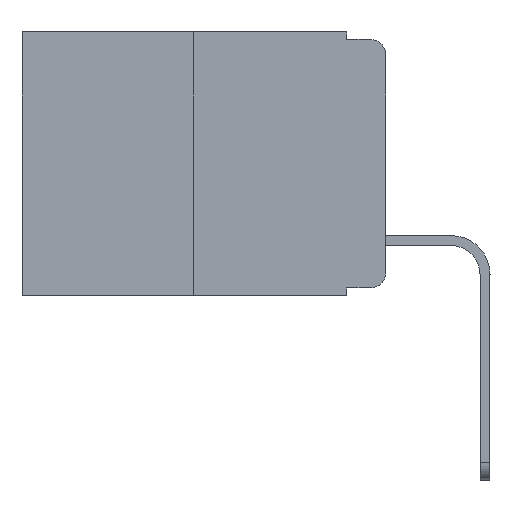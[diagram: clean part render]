
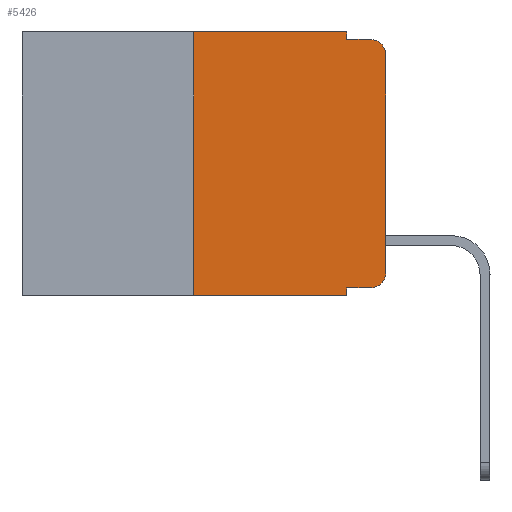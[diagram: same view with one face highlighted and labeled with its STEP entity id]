
A CAD part, left-side view. The second image highlights one B-rep face of the part: STEP entity #5426.
In plain terms, the highlighted planar face has unit normal (-1, 0, 0).
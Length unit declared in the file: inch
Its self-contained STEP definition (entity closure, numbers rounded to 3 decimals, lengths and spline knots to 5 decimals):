
#352 = VERTEX_POINT ( 'NONE', #11392 ) ;
#611 = DIRECTION ( 'NONE',  ( 0., 0., -1. ) ) ;
#621 = EDGE_CURVE ( 'NONE', #10920, #8780, #8117, .T. ) ;
#661 = VECTOR ( 'NONE', #7831, 39.37008 ) ;
#679 = DIRECTION ( 'NONE',  ( 0., 0., -1. ) ) ;
#729 = LINE ( 'NONE', #7810, #7426 ) ;
#863 = DIRECTION ( 'NONE',  ( 0., 0., -1. ) ) ;
#1055 = VERTEX_POINT ( 'NONE', #1663 ) ;
#1110 = ORIENTED_EDGE ( 'NONE', *, *, #11555, .T. ) ;
#1225 = CARTESIAN_POINT ( 'NONE',  ( 0., 0.473, 0. ) ) ;
#1227 = LINE ( 'NONE', #2138, #4111 ) ;
#1252 = ORIENTED_EDGE ( 'NONE', *, *, #7644, .T. ) ;
#1360 = ORIENTED_EDGE ( 'NONE', *, *, #11955, .F. ) ;
#1390 = CIRCLE ( 'NONE', #7680, 0.02 ) ;
#1627 = VECTOR ( 'NONE', #9238, 39.37008 ) ;
#1663 = CARTESIAN_POINT ( 'NONE',  ( 0., 0., -0.03 ) ) ;
#1911 = EDGE_CURVE ( 'NONE', #1055, #9202, #5476, .T. ) ;
#2065 = DIRECTION ( 'NONE',  ( 0., 0., 1. ) ) ;
#2138 = CARTESIAN_POINT ( 'NONE',  ( 0., 0., 0. ) ) ;
#2161 = CARTESIAN_POINT ( 'NONE',  ( 0., 0.02, -0.01 ) ) ;
#2616 = ORIENTED_EDGE ( 'NONE', *, *, #5266, .F. ) ;
#2646 = LINE ( 'NONE', #10412, #11931 ) ;
#3021 = PLANE ( 'NONE',  #4614 ) ;
#3123 = FACE_OUTER_BOUND ( 'NONE', #6134, .T. ) ;
#3201 = CARTESIAN_POINT ( 'NONE',  ( 0., 0.02, -0.333 ) ) ;
#3564 = CARTESIAN_POINT ( 'NONE',  ( 0., 0.051, -0.01 ) ) ;
#3693 = VECTOR ( 'NONE', #863, 39.37008 ) ;
#3713 = DIRECTION ( 'NONE',  ( 0., -1., 0. ) ) ;
#3985 = DIRECTION ( 'NONE',  ( 1., 0., 0. ) ) ;
#4042 = EDGE_CURVE ( 'NONE', #11896, #6898, #8013, .T. ) ;
#4111 = VECTOR ( 'NONE', #10077, 39.37008 ) ;
#4382 = ORIENTED_EDGE ( 'NONE', *, *, #621, .F. ) ;
#4486 = CARTESIAN_POINT ( 'NONE',  ( 0., 0.02, -0.313 ) ) ;
#4570 = VERTEX_POINT ( 'NONE', #8817 ) ;
#4582 = DIRECTION ( 'NONE',  ( 0., -1., 0. ) ) ;
#4604 = CARTESIAN_POINT ( 'NONE',  ( 0., 0.02, -0.03 ) ) ;
#4614 = AXIS2_PLACEMENT_3D ( 'NONE', #1225, #3985, #10744 ) ;
#4845 = CARTESIAN_POINT ( 'NONE',  ( 0., 0.051, 0. ) ) ;
#5214 = ORIENTED_EDGE ( 'NONE', *, *, #5924, .T. ) ;
#5266 = EDGE_CURVE ( 'NONE', #8780, #9202, #6140, .T. ) ;
#5426 = ADVANCED_FACE ( 'NONE', ( #3123 ), #3021, .F. ) ;
#5476 = CIRCLE ( 'NONE', #7313, 0.02 ) ;
#5506 = ORIENTED_EDGE ( 'NONE', *, *, #1911, .T. ) ;
#5924 = EDGE_CURVE ( 'NONE', #11896, #352, #2646, .T. ) ;
#5969 = CARTESIAN_POINT ( 'NONE',  ( 0., 0.051, 0. ) ) ;
#6134 = EDGE_LOOP ( 'NONE', ( #10875, #5506, #2616, #4382, #1360, #12085, #5214, #11938, #1110, #1252 ) ) ;
#6140 = LINE ( 'NONE', #3564, #661 ) ;
#6372 = DIRECTION ( 'NONE',  ( -1., 0., 0. ) ) ;
#6440 = DIRECTION ( 'NONE',  ( -1., 0., 0. ) ) ;
#6471 = VECTOR ( 'NONE', #2065, 39.37008 ) ;
#6796 = EDGE_CURVE ( 'NONE', #4570, #1055, #1227, .T. ) ;
#6825 = VERTEX_POINT ( 'NONE', #7967 ) ;
#6898 = VERTEX_POINT ( 'NONE', #10285 ) ;
#7241 = CARTESIAN_POINT ( 'NONE',  ( 0., 0.051, -0.01 ) ) ;
#7313 = AXIS2_PLACEMENT_3D ( 'NONE', #4604, #6372, #679 ) ;
#7426 = VECTOR ( 'NONE', #7978, 39.37008 ) ;
#7644 = EDGE_CURVE ( 'NONE', #12211, #4570, #1390, .T. ) ;
#7680 = AXIS2_PLACEMENT_3D ( 'NONE', #4486, #6440, #611 ) ;
#7810 = CARTESIAN_POINT ( 'NONE',  ( 0., 0.051, -0.333 ) ) ;
#7831 = DIRECTION ( 'NONE',  ( 0., -1., 0. ) ) ;
#7883 = VECTOR ( 'NONE', #3713, 39.37008 ) ;
#7967 = CARTESIAN_POINT ( 'NONE',  ( 0., 0.051, -0.333 ) ) ;
#7978 = DIRECTION ( 'NONE',  ( 0., -1., 0. ) ) ;
#8013 = LINE ( 'NONE', #11863, #6471 ) ;
#8117 = LINE ( 'NONE', #4845, #3693 ) ;
#8184 = LINE ( 'NONE', #12408, #7883 ) ;
#8780 = VERTEX_POINT ( 'NONE', #7241 ) ;
#8817 = CARTESIAN_POINT ( 'NONE',  ( 0., 0., -0.313 ) ) ;
#9202 = VERTEX_POINT ( 'NONE', #2161 ) ;
#9238 = DIRECTION ( 'NONE',  ( 0., 0., -1. ) ) ;
#9383 = CARTESIAN_POINT ( 'NONE',  ( 0., 0.25, -0.343 ) ) ;
#10077 = DIRECTION ( 'NONE',  ( 0., 0., 1. ) ) ;
#10285 = CARTESIAN_POINT ( 'NONE',  ( 0., 0.25, 0. ) ) ;
#10412 = CARTESIAN_POINT ( 'NONE',  ( 0., 0.473, -0.343 ) ) ;
#10744 = DIRECTION ( 'NONE',  ( 0., 0., -1. ) ) ;
#10875 = ORIENTED_EDGE ( 'NONE', *, *, #6796, .T. ) ;
#10920 = VERTEX_POINT ( 'NONE', #5969 ) ;
#11055 = LINE ( 'NONE', #11405, #1627 ) ;
#11392 = CARTESIAN_POINT ( 'NONE',  ( 0., 0.051, -0.343 ) ) ;
#11405 = CARTESIAN_POINT ( 'NONE',  ( 0., 0.051, 0. ) ) ;
#11555 = EDGE_CURVE ( 'NONE', #6825, #12211, #729, .T. ) ;
#11863 = CARTESIAN_POINT ( 'NONE',  ( 0., 0.25, 0. ) ) ;
#11896 = VERTEX_POINT ( 'NONE', #9383 ) ;
#11931 = VECTOR ( 'NONE', #4582, 39.37008 ) ;
#11938 = ORIENTED_EDGE ( 'NONE', *, *, #12419, .F. ) ;
#11955 = EDGE_CURVE ( 'NONE', #6898, #10920, #8184, .T. ) ;
#12085 = ORIENTED_EDGE ( 'NONE', *, *, #4042, .F. ) ;
#12211 = VERTEX_POINT ( 'NONE', #3201 ) ;
#12408 = CARTESIAN_POINT ( 'NONE',  ( 0., 0.473, 0. ) ) ;
#12419 = EDGE_CURVE ( 'NONE', #6825, #352, #11055, .T. ) ;
